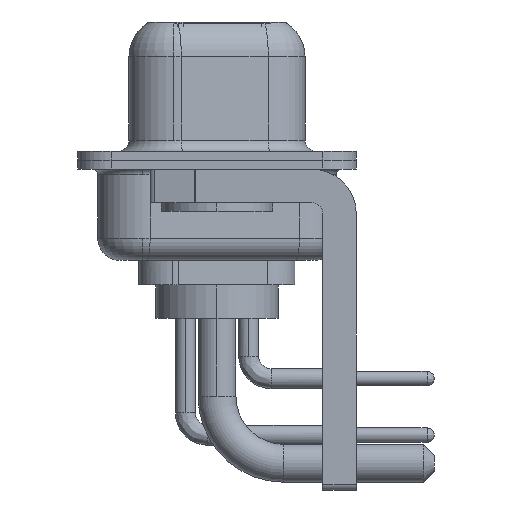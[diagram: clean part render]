
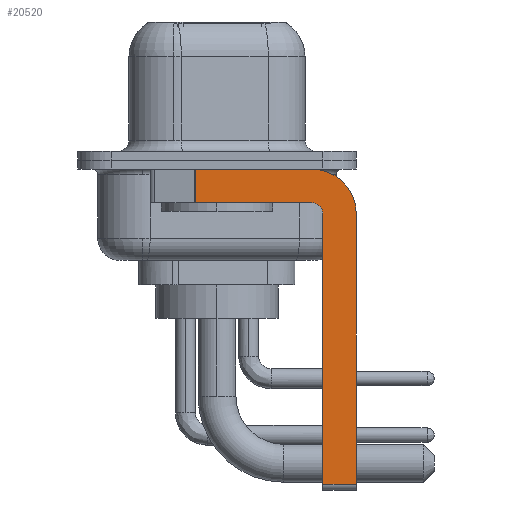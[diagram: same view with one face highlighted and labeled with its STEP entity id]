
A CAD part, left-side view. The second image highlights one B-rep face of the part: STEP entity #20520.
In plain terms, the highlighted planar face has unit normal (-1, 0, 0).
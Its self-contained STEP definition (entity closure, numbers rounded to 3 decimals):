
#413 = DIRECTION ( 'NONE',  ( 1., 0., 0. ) ) ;
#582 = CARTESIAN_POINT ( 'NONE',  ( -2.9, -6.25, -14.55 ) ) ;
#925 = ORIENTED_EDGE ( 'NONE', *, *, #4919, .F. ) ;
#1134 = DIRECTION ( 'NONE',  ( 0., 0., -1. ) ) ;
#1313 = CIRCLE ( 'NONE', #19124, 0.5 ) ;
#2418 = CARTESIAN_POINT ( 'NONE',  ( -2.9, -4.75, -2.4 ) ) ;
#2781 = VECTOR ( 'NONE', #16853, 1000. ) ;
#2822 = VERTEX_POINT ( 'NONE', #19442 ) ;
#2881 = LINE ( 'NONE', #19395, #13087 ) ;
#3279 = CARTESIAN_POINT ( 'NONE',  ( -2.9, -4.25, -1.9 ) ) ;
#3716 = EDGE_CURVE ( 'NONE', #10430, #5199, #14492, .T. ) ;
#3897 = CIRCLE ( 'NONE', #14397, 2. ) ;
#4289 = EDGE_CURVE ( 'NONE', #10430, #11679, #9755, .T. ) ;
#4636 = CARTESIAN_POINT ( 'NONE',  ( -2.9, -4.75, -14.8 ) ) ;
#4723 = LINE ( 'NONE', #6472, #18882 ) ;
#4824 = VECTOR ( 'NONE', #16018, 1000. ) ;
#4885 = DIRECTION ( 'NONE',  ( 1., 0., 0. ) ) ;
#4919 = EDGE_CURVE ( 'NONE', #5199, #7040, #1313, .T. ) ;
#5138 = LINE ( 'NONE', #3279, #2781 ) ;
#5199 = VERTEX_POINT ( 'NONE', #2418 ) ;
#6450 = VERTEX_POINT ( 'NONE', #12507 ) ;
#6472 = CARTESIAN_POINT ( 'NONE',  ( -2.9, 3., -0.4 ) ) ;
#6477 = CARTESIAN_POINT ( 'NONE',  ( -2.9, -4.75, -14.55 ) ) ;
#6698 = DIRECTION ( 'NONE',  ( 0., 0., 1. ) ) ;
#6735 = EDGE_CURVE ( 'NONE', #7040, #6450, #5138, .T. ) ;
#6737 = DIRECTION ( 'NONE',  ( 0., 0., -1. ) ) ;
#6888 = DIRECTION ( 'NONE',  ( 0., 0., -1. ) ) ;
#7027 = CARTESIAN_POINT ( 'NONE',  ( -2.9, -4.25, -2.4 ) ) ;
#7040 = VERTEX_POINT ( 'NONE', #13013 ) ;
#7067 = ORIENTED_EDGE ( 'NONE', *, *, #4289, .T. ) ;
#7708 = LINE ( 'NONE', #16137, #19718 ) ;
#7826 = EDGE_CURVE ( 'NONE', #13237, #2822, #4723, .T. ) ;
#8288 = EDGE_LOOP ( 'NONE', ( #12346, #19767, #19189, #925, #21196, #7067, #16229, #20357 ) ) ;
#9566 = DIRECTION ( 'NONE',  ( 0., 0., -1. ) ) ;
#9755 = LINE ( 'NONE', #16420, #19797 ) ;
#10127 = EDGE_CURVE ( 'NONE', #2822, #20126, #3897, .T. ) ;
#10430 = VERTEX_POINT ( 'NONE', #6477 ) ;
#10665 = CARTESIAN_POINT ( 'NONE',  ( -2.9, -6.25, -2.4 ) ) ;
#11505 = AXIS2_PLACEMENT_3D ( 'NONE', #20213, #413, #6888 ) ;
#11679 = VERTEX_POINT ( 'NONE', #582 ) ;
#12346 = ORIENTED_EDGE ( 'NONE', *, *, #7826, .F. ) ;
#12507 = CARTESIAN_POINT ( 'NONE',  ( -2.9, 0.978, -1.9 ) ) ;
#12791 = EDGE_CURVE ( 'NONE', #13237, #6450, #7708, .T. ) ;
#13013 = CARTESIAN_POINT ( 'NONE',  ( -2.9, -4.25, -1.9 ) ) ;
#13087 = VECTOR ( 'NONE', #9566, 1000. ) ;
#13237 = VERTEX_POINT ( 'NONE', #17865 ) ;
#13710 = DIRECTION ( 'NONE',  ( -1., 0., 0. ) ) ;
#14397 = AXIS2_PLACEMENT_3D ( 'NONE', #18430, #4885, #6737 ) ;
#14492 = LINE ( 'NONE', #4636, #4824 ) ;
#14952 = EDGE_CURVE ( 'NONE', #20126, #11679, #2881, .T. ) ;
#16018 = DIRECTION ( 'NONE',  ( 0., 0., 1. ) ) ;
#16137 = CARTESIAN_POINT ( 'NONE',  ( -2.9, 0.978, -1.9 ) ) ;
#16229 = ORIENTED_EDGE ( 'NONE', *, *, #14952, .F. ) ;
#16420 = CARTESIAN_POINT ( 'NONE',  ( -2.9, -4.25, -14.55 ) ) ;
#16853 = DIRECTION ( 'NONE',  ( 0., 1., 0. ) ) ;
#17865 = CARTESIAN_POINT ( 'NONE',  ( -2.9, 0.978, -0.4 ) ) ;
#18430 = CARTESIAN_POINT ( 'NONE',  ( -2.9, -4.25, -2.4 ) ) ;
#18693 = PLANE ( 'NONE',  #11505 ) ;
#18882 = VECTOR ( 'NONE', #21424, 1000. ) ;
#19124 = AXIS2_PLACEMENT_3D ( 'NONE', #7027, #13710, #6698 ) ;
#19189 = ORIENTED_EDGE ( 'NONE', *, *, #6735, .F. ) ;
#19395 = CARTESIAN_POINT ( 'NONE',  ( -2.9, -6.25, -2.4 ) ) ;
#19442 = CARTESIAN_POINT ( 'NONE',  ( -2.9, -4.25, -0.4 ) ) ;
#19718 = VECTOR ( 'NONE', #1134, 1000. ) ;
#19767 = ORIENTED_EDGE ( 'NONE', *, *, #12791, .T. ) ;
#19797 = VECTOR ( 'NONE', #21529, 1000. ) ;
#20126 = VERTEX_POINT ( 'NONE', #10665 ) ;
#20213 = CARTESIAN_POINT ( 'NONE',  ( -2.9, -4.25, -2.4 ) ) ;
#20324 = FACE_OUTER_BOUND ( 'NONE', #8288, .T. ) ;
#20357 = ORIENTED_EDGE ( 'NONE', *, *, #10127, .F. ) ;
#20520 = ADVANCED_FACE ( 'NONE', ( #20324 ), #18693, .F. ) ;
#21196 = ORIENTED_EDGE ( 'NONE', *, *, #3716, .F. ) ;
#21424 = DIRECTION ( 'NONE',  ( 0., -1., 0. ) ) ;
#21529 = DIRECTION ( 'NONE',  ( 0., -1., 0. ) ) ;
